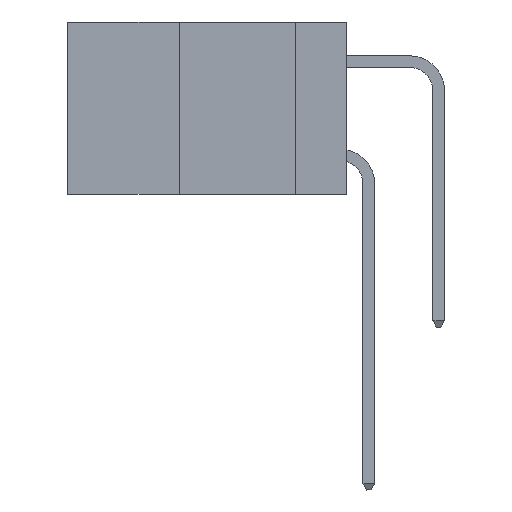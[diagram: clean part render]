
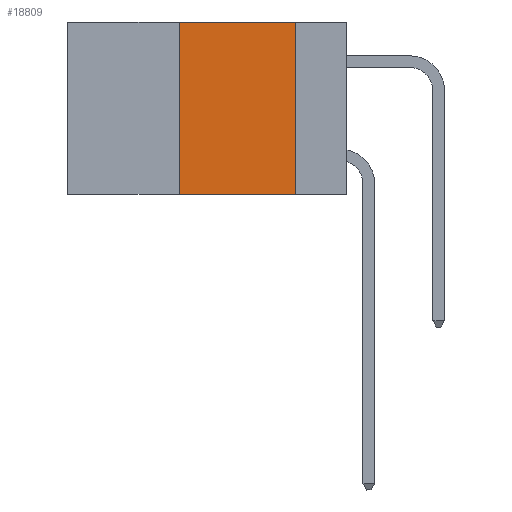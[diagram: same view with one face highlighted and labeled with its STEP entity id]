
A CAD part, left-side view. The second image highlights one B-rep face of the part: STEP entity #18809.
In plain terms, the highlighted planar face has unit normal (-1, 0, 0).
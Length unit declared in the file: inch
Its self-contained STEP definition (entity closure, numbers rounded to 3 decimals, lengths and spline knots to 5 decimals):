
#1802 = CARTESIAN_POINT ( 'NONE',  ( 0., 0.36, 0. ) ) ;
#2246 = VERTEX_POINT ( 'NONE', #1802 ) ;
#3516 = VECTOR ( 'NONE', #12496, 39.37008 ) ;
#6845 = CARTESIAN_POINT ( 'NONE',  ( 0., 0.11, 0. ) ) ;
#6983 = CARTESIAN_POINT ( 'NONE',  ( 0., 0.6, -0.37 ) ) ;
#7627 = PLANE ( 'NONE',  #24739 ) ;
#7660 = DIRECTION ( 'NONE',  ( 0., 0., -1. ) ) ;
#7718 = DIRECTION ( 'NONE',  ( 1., 0., 0. ) ) ;
#8500 = VECTOR ( 'NONE', #9153, 39.37008 ) ;
#9131 = VECTOR ( 'NONE', #7660, 39.37008 ) ;
#9153 = DIRECTION ( 'NONE',  ( 0., -1., 0. ) ) ;
#9298 = VERTEX_POINT ( 'NONE', #22624 ) ;
#9368 = VERTEX_POINT ( 'NONE', #6845 ) ;
#11627 = CARTESIAN_POINT ( 'NONE',  ( 0., 0.6, 0. ) ) ;
#11665 = CARTESIAN_POINT ( 'NONE',  ( 0., 0.11, 0. ) ) ;
#12496 = DIRECTION ( 'NONE',  ( 0., 0., 1. ) ) ;
#12507 = VERTEX_POINT ( 'NONE', #17477 ) ;
#13217 = EDGE_CURVE ( 'NONE', #12507, #2246, #20694, .T. ) ;
#13273 = LINE ( 'NONE', #6983, #8500 ) ;
#14178 = ORIENTED_EDGE ( 'NONE', *, *, #18185, .F. ) ;
#15378 = EDGE_CURVE ( 'NONE', #12507, #9298, #13273, .T. ) ;
#16096 = DIRECTION ( 'NONE',  ( 0., -1., 0. ) ) ;
#16289 = CARTESIAN_POINT ( 'NONE',  ( 0., 0.36, 0. ) ) ;
#16405 = LINE ( 'NONE', #11665, #9131 ) ;
#16954 = ORIENTED_EDGE ( 'NONE', *, *, #13217, .F. ) ;
#16992 = FACE_OUTER_BOUND ( 'NONE', #17318, .T. ) ;
#17318 = EDGE_LOOP ( 'NONE', ( #21797, #14178, #16954, #21056 ) ) ;
#17477 = CARTESIAN_POINT ( 'NONE',  ( 0., 0.36, -0.37 ) ) ;
#18100 = EDGE_CURVE ( 'NONE', #9368, #9298, #16405, .T. ) ;
#18185 = EDGE_CURVE ( 'NONE', #2246, #9368, #21216, .T. ) ;
#18809 = ADVANCED_FACE ( 'NONE', ( #16992 ), #7627, .F. ) ;
#19271 = VECTOR ( 'NONE', #16096, 39.37008 ) ;
#20694 = LINE ( 'NONE', #16289, #3516 ) ;
#21056 = ORIENTED_EDGE ( 'NONE', *, *, #15378, .T. ) ;
#21216 = LINE ( 'NONE', #26135, #19271 ) ;
#21797 = ORIENTED_EDGE ( 'NONE', *, *, #18100, .F. ) ;
#22624 = CARTESIAN_POINT ( 'NONE',  ( 0., 0.11, -0.37 ) ) ;
#23964 = DIRECTION ( 'NONE',  ( 0., 0., -1. ) ) ;
#24739 = AXIS2_PLACEMENT_3D ( 'NONE', #11627, #7718, #23964 ) ;
#26135 = CARTESIAN_POINT ( 'NONE',  ( 0., 0.6, 0. ) ) ;
